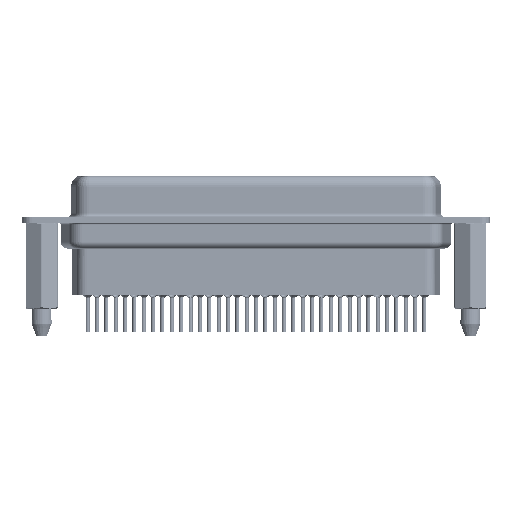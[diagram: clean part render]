
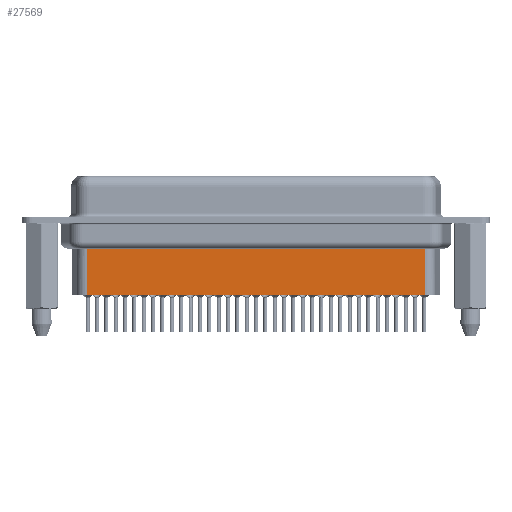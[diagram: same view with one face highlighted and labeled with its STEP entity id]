
A CAD part, front view. The second image highlights one B-rep face of the part: STEP entity #27569.
In plain terms, the highlighted planar face has unit normal (0, -1, 0).
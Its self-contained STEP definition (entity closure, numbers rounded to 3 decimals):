
#1730 = VECTOR ( 'NONE', #10078, 1000. ) ;
#2153 = AXIS2_PLACEMENT_3D ( 'NONE', #13142, #17938, #15544 ) ;
#4562 = CARTESIAN_POINT ( 'NONE',  ( 56.794, -3.5, -3.1 ) ) ;
#5656 = CARTESIAN_POINT ( 'NONE',  ( 56.794, -3.5, -4.097 ) ) ;
#6620 = VECTOR ( 'NONE', #24969, 1000. ) ;
#7101 = CARTESIAN_POINT ( 'NONE',  ( 6.706, -3.5, -11.15 ) ) ;
#9201 = EDGE_LOOP ( 'NONE', ( #29985, #9381, #30243, #11411 ) ) ;
#9381 = ORIENTED_EDGE ( 'NONE', *, *, #30880, .T. ) ;
#10078 = DIRECTION ( 'NONE',  ( -1., 0., 0. ) ) ;
#11411 = ORIENTED_EDGE ( 'NONE', *, *, #13057, .F. ) ;
#11440 = CARTESIAN_POINT ( 'NONE',  ( 56.794, -3.5, -11.15 ) ) ;
#13057 = EDGE_CURVE ( 'NONE', #28541, #20269, #30559, .T. ) ;
#13136 = EDGE_CURVE ( 'NONE', #26576, #20269, #20312, .T. ) ;
#13142 = CARTESIAN_POINT ( 'NONE',  ( 6.706, -3.5, -3.1 ) ) ;
#14542 = LINE ( 'NONE', #4562, #6620 ) ;
#15544 = DIRECTION ( 'NONE',  ( 1., 0., 0. ) ) ;
#15797 = VECTOR ( 'NONE', #33487, 1000. ) ;
#16086 = EDGE_CURVE ( 'NONE', #31671, #28541, #14542, .T. ) ;
#17296 = LINE ( 'NONE', #22951, #1730 ) ;
#17938 = DIRECTION ( 'NONE',  ( 0., -1., 0. ) ) ;
#20269 = VERTEX_POINT ( 'NONE', #23954 ) ;
#20312 = LINE ( 'NONE', #28873, #15797 ) ;
#21024 = PLANE ( 'NONE',  #2153 ) ;
#21502 = VECTOR ( 'NONE', #28022, 1000. ) ;
#22951 = CARTESIAN_POINT ( 'NONE',  ( 6.459, -3.5, -4.097 ) ) ;
#23180 = CARTESIAN_POINT ( 'NONE',  ( 6.706, -3.5, -4.097 ) ) ;
#23954 = CARTESIAN_POINT ( 'NONE',  ( 6.706, -3.5, -11.15 ) ) ;
#24969 = DIRECTION ( 'NONE',  ( 0., 0., -1. ) ) ;
#26576 = VERTEX_POINT ( 'NONE', #23180 ) ;
#27569 = ADVANCED_FACE ( 'NONE', ( #28558 ), #21024, .T. ) ;
#28022 = DIRECTION ( 'NONE',  ( -1., 0., 0. ) ) ;
#28541 = VERTEX_POINT ( 'NONE', #11440 ) ;
#28558 = FACE_OUTER_BOUND ( 'NONE', #9201, .T. ) ;
#28873 = CARTESIAN_POINT ( 'NONE',  ( 6.706, -3.5, -3.1 ) ) ;
#29985 = ORIENTED_EDGE ( 'NONE', *, *, #16086, .F. ) ;
#30243 = ORIENTED_EDGE ( 'NONE', *, *, #13136, .T. ) ;
#30559 = LINE ( 'NONE', #7101, #21502 ) ;
#30880 = EDGE_CURVE ( 'NONE', #31671, #26576, #17296, .T. ) ;
#31671 = VERTEX_POINT ( 'NONE', #5656 ) ;
#33487 = DIRECTION ( 'NONE',  ( 0., 0., -1. ) ) ;
